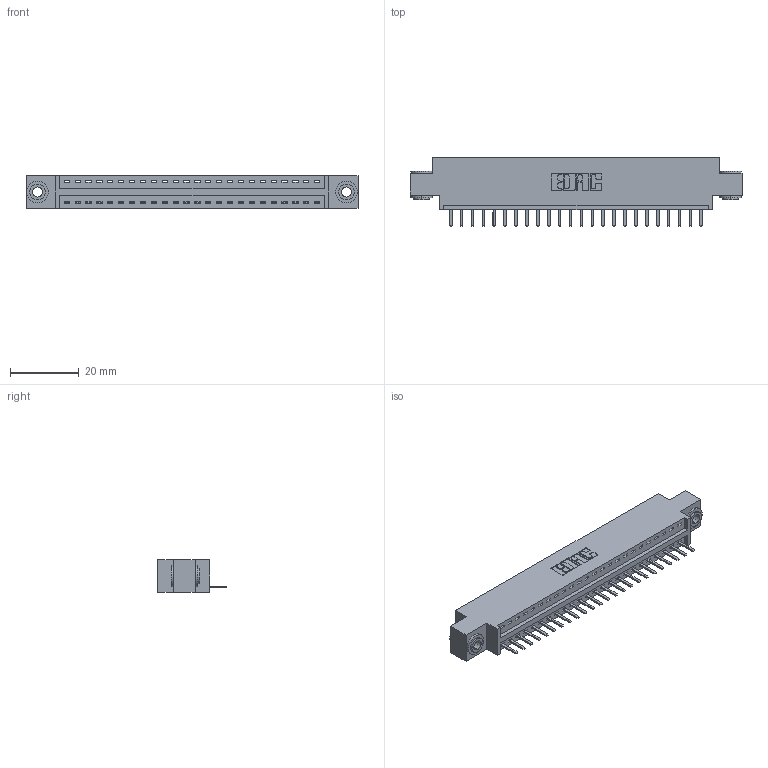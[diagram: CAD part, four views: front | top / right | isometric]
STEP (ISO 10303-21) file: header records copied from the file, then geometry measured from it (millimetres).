
FILE_DESCRIPTION (( 'STEP AP203' ), '1' );
FILE_NAME ('346-024-520-603.STEP', '2022-05-05T22:23:03', ( '' ), ( '' ), 'SwSTEP 2.0', 'SolidWorks 2020', '' );
FILE_SCHEMA (( 'CONFIG_CONTROL_DESIGN' ));
Length unit declared in the file: inch
Products named in the file (4): 346-024-520-603; 345-250-002_345-250-002-102; 345-292-001_345-293-120; 346 Part_0.170 Offset - 0.156 Dia-TH
Assembly tree (27 placements, depth 2):
  346-024-520-603
    346 Part_0.170 Offset - 0.156 Dia-TH
    345-292-001_345-293-120  x24
    345-250-002_345-250-002-102  x2
Bounding box: 96.77 x 20.02 x 9.4 mm (x, y, z)
Volume: 8917 mm3; surface area: 11132.3 mm2
Topology: 27 solids, 27 shells, 1666 faces, 4869 edges, 3178 vertices
Faces by surface type: plane 1112, cylinder 546, cone 8
Entity records: 18630 total; most frequent: CARTESIAN_POINT 3193, ORIENTED_EDGE 3130, DIRECTION 2855, EDGE_CURVE 1565, VECTOR 1309, LINE 1309, VERTEX_POINT 1038, AXIS2_PLACEMENT_3D 773
